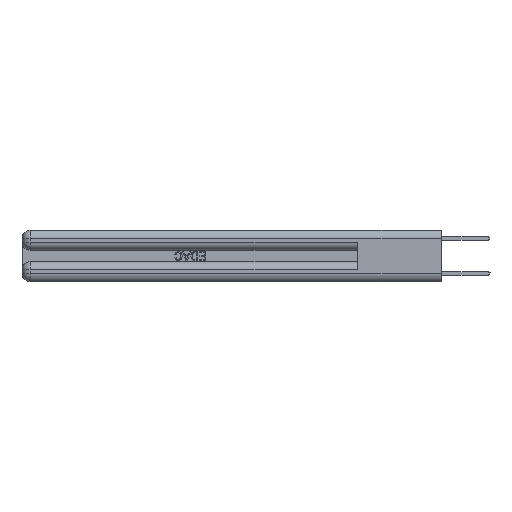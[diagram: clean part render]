
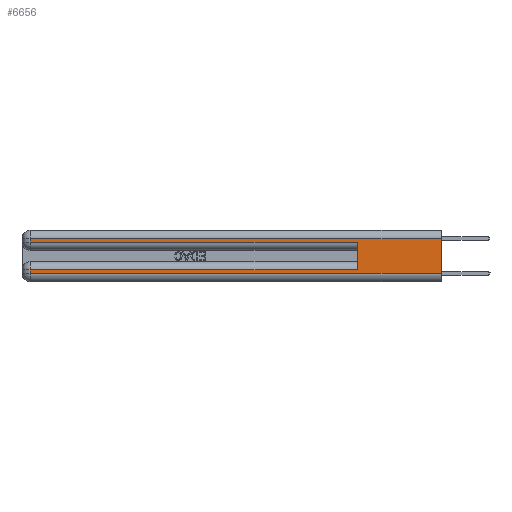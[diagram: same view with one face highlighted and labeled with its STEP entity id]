
A CAD part, left-side view. The second image highlights one B-rep face of the part: STEP entity #6656.
In plain terms, the highlighted planar face has unit normal (-1, 0, 0).
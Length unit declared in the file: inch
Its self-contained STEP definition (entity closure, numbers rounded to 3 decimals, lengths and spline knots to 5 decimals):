
#498 = EDGE_LOOP ( 'NONE', ( #10901, #22130, #6166, #13129, #18005, #31792, #11123, #22901 ) ) ;
#656 = VERTEX_POINT ( 'NONE', #24321 ) ;
#795 = CARTESIAN_POINT ( 'NONE',  ( 0., 0., 0.37 ) ) ;
#1037 = CARTESIAN_POINT ( 'NONE',  ( 0., 2.94, 0.085 ) ) ;
#2181 = CARTESIAN_POINT ( 'NONE',  ( 0., 0.6, 0.085 ) ) ;
#2543 = CARTESIAN_POINT ( 'NONE',  ( 0., 0., 0.06 ) ) ;
#2556 = VECTOR ( 'NONE', #12882, 39.37008 ) ;
#3259 = EDGE_CURVE ( 'NONE', #4768, #23388, #31243, .T. ) ;
#3591 = FACE_OUTER_BOUND ( 'NONE', #498, .T. ) ;
#4042 = VERTEX_POINT ( 'NONE', #22000 ) ;
#4278 = EDGE_CURVE ( 'NONE', #656, #24837, #4708, .T. ) ;
#4324 = CARTESIAN_POINT ( 'NONE',  ( 0., 2.94, 0.285 ) ) ;
#4400 = VECTOR ( 'NONE', #26084, 39.37008 ) ;
#4708 = LINE ( 'NONE', #795, #23945 ) ;
#4768 = VERTEX_POINT ( 'NONE', #2181 ) ;
#6166 = ORIENTED_EDGE ( 'NONE', *, *, #32670, .T. ) ;
#6656 = ADVANCED_FACE ( 'NONE', ( #3591 ), #21563, .F. ) ;
#7410 = CARTESIAN_POINT ( 'NONE',  ( 0., 0.6, 0.145 ) ) ;
#7539 = VECTOR ( 'NONE', #20531, 39.37008 ) ;
#7894 = VERTEX_POINT ( 'NONE', #24495 ) ;
#8305 = DIRECTION ( 'NONE',  ( 0., 0., -1. ) ) ;
#9954 = LINE ( 'NONE', #30736, #7539 ) ;
#9994 = CARTESIAN_POINT ( 'NONE',  ( 0., 0., 0.085 ) ) ;
#10761 = CARTESIAN_POINT ( 'NONE',  ( 0., 0., 0.285 ) ) ;
#10901 = ORIENTED_EDGE ( 'NONE', *, *, #4278, .F. ) ;
#11123 = ORIENTED_EDGE ( 'NONE', *, *, #16855, .T. ) ;
#12380 = CARTESIAN_POINT ( 'NONE',  ( 0., 2.94, 0.06 ) ) ;
#12757 = DIRECTION ( 'NONE',  ( 0., 0., 1. ) ) ;
#12882 = DIRECTION ( 'NONE',  ( 0., -1., 0. ) ) ;
#13129 = ORIENTED_EDGE ( 'NONE', *, *, #32377, .T. ) ;
#15218 = CARTESIAN_POINT ( 'NONE',  ( 0., 2.94, 0.37 ) ) ;
#16627 = DIRECTION ( 'NONE',  ( 0., 0., -1. ) ) ;
#16855 = EDGE_CURVE ( 'NONE', #23388, #20661, #27212, .T. ) ;
#16954 = DIRECTION ( 'NONE',  ( 1., 0., 0. ) ) ;
#17548 = EDGE_CURVE ( 'NONE', #20661, #24837, #9954, .T. ) ;
#17789 = DIRECTION ( 'NONE',  ( 0., 0., -1. ) ) ;
#17975 = LINE ( 'NONE', #7410, #20716 ) ;
#18005 = ORIENTED_EDGE ( 'NONE', *, *, #28822, .F. ) ;
#19264 = LINE ( 'NONE', #20992, #20042 ) ;
#20042 = VECTOR ( 'NONE', #31193, 39.37008 ) ;
#20531 = DIRECTION ( 'NONE',  ( 0., -1., 0. ) ) ;
#20661 = VERTEX_POINT ( 'NONE', #12380 ) ;
#20716 = VECTOR ( 'NONE', #12757, 39.37008 ) ;
#20992 = CARTESIAN_POINT ( 'NONE',  ( 0., 0., 0.31 ) ) ;
#21563 = PLANE ( 'NONE',  #29592 ) ;
#22000 = CARTESIAN_POINT ( 'NONE',  ( 0., 0.6, 0.285 ) ) ;
#22130 = ORIENTED_EDGE ( 'NONE', *, *, #26886, .T. ) ;
#22901 = ORIENTED_EDGE ( 'NONE', *, *, #17548, .T. ) ;
#23388 = VERTEX_POINT ( 'NONE', #1037 ) ;
#23945 = VECTOR ( 'NONE', #8305, 39.37008 ) ;
#24321 = CARTESIAN_POINT ( 'NONE',  ( 0., 0., 0.31 ) ) ;
#24495 = CARTESIAN_POINT ( 'NONE',  ( 0., 2.94, 0.31 ) ) ;
#24552 = VECTOR ( 'NONE', #32247, 39.37008 ) ;
#24776 = CARTESIAN_POINT ( 'NONE',  ( 0., 0., 0.37 ) ) ;
#24837 = VERTEX_POINT ( 'NONE', #2543 ) ;
#26084 = DIRECTION ( 'NONE',  ( 0., 1., 0. ) ) ;
#26789 = VECTOR ( 'NONE', #17789, 39.37008 ) ;
#26886 = EDGE_CURVE ( 'NONE', #656, #7894, #19264, .T. ) ;
#27212 = LINE ( 'NONE', #15218, #26789 ) ;
#27341 = LINE ( 'NONE', #29680, #24552 ) ;
#28822 = EDGE_CURVE ( 'NONE', #4768, #4042, #17975, .T. ) ;
#29592 = AXIS2_PLACEMENT_3D ( 'NONE', #24776, #16954, #16627 ) ;
#29680 = CARTESIAN_POINT ( 'NONE',  ( 0., 2.94, 0.37 ) ) ;
#29980 = VERTEX_POINT ( 'NONE', #4324 ) ;
#30736 = CARTESIAN_POINT ( 'NONE',  ( 0., 0., 0.06 ) ) ;
#31193 = DIRECTION ( 'NONE',  ( 0., 1., 0. ) ) ;
#31243 = LINE ( 'NONE', #9994, #4400 ) ;
#31792 = ORIENTED_EDGE ( 'NONE', *, *, #3259, .T. ) ;
#31803 = LINE ( 'NONE', #10761, #2556 ) ;
#32247 = DIRECTION ( 'NONE',  ( 0., 0., -1. ) ) ;
#32377 = EDGE_CURVE ( 'NONE', #29980, #4042, #31803, .T. ) ;
#32670 = EDGE_CURVE ( 'NONE', #7894, #29980, #27341, .T. ) ;
